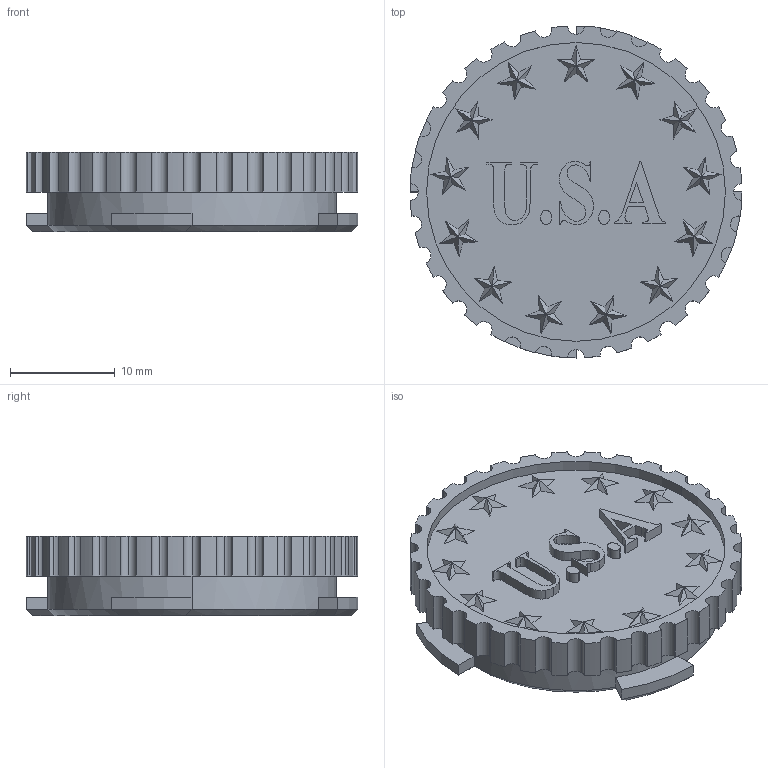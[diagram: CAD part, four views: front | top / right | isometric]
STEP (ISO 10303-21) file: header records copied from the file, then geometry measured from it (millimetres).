
FILE_DESCRIPTION (( 'STEP AP203' ), '1' );
FILE_NAME ('AF-HF-TK-PRT-005-STEP_USA.STEP', '2020-12-04T14:11:05', ( '' ), ( '' ), 'SwSTEP 2.0', 'SolidWorks 2018', '' );
FILE_SCHEMA (( 'CONFIG_CONTROL_DESIGN' ));
Length unit declared in the file: inch
Products named in the file (1): AF-HF-TK-PRT-005-STEP_USA
Bounding box: 31.75 x 31.75 x 7.62 mm (x, y, z)
Volume: 3704 mm3; surface area: 2772.9 mm2
Topology: 1 solids, 1 shells, 359 faces, 981 edges, 646 vertices
Faces by surface type: plane 207, cylinder 89, bspline 48, cone 13, sphere 2
Entity records: 13185 total; most frequent: CARTESIAN_POINT 4179, ORIENTED_EDGE 1962, DIRECTION 1692, EDGE_CURVE 981, LINE 670, VECTOR 670, VERTEX_POINT 646, AXIS2_PLACEMENT_3D 511
